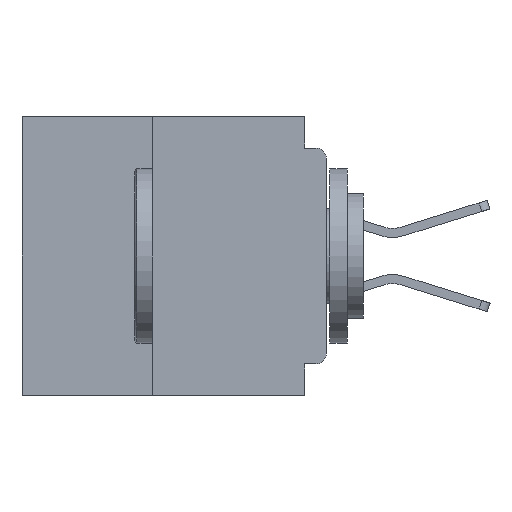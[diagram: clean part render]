
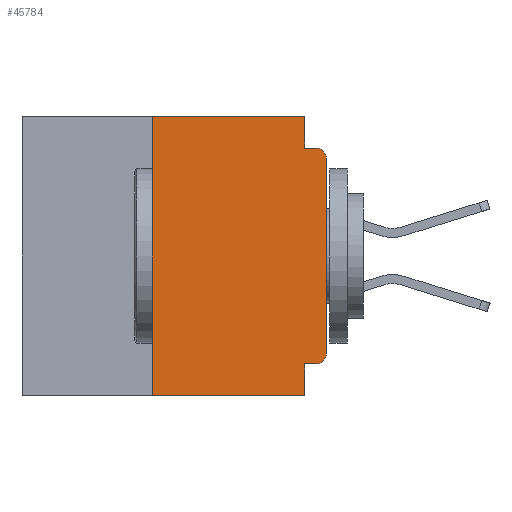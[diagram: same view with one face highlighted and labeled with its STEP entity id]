
A CAD part, left-side view. The second image highlights one B-rep face of the part: STEP entity #45784.
In plain terms, the highlighted planar face has unit normal (-1, 0, 0).
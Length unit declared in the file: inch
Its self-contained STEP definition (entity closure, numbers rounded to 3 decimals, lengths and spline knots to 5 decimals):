
#815 = VERTEX_POINT ( 'NONE', #24449 ) ;
#2517 = PLANE ( 'NONE',  #50532 ) ;
#2631 = CARTESIAN_POINT ( 'NONE',  ( 0., 0.437, 0. ) ) ;
#3236 = ORIENTED_EDGE ( 'NONE', *, *, #13706, .T. ) ;
#3609 = ORIENTED_EDGE ( 'NONE', *, *, #6461, .T. ) ;
#6225 = CARTESIAN_POINT ( 'NONE',  ( 0., 0.031, -0.355 ) ) ;
#6461 = EDGE_CURVE ( 'NONE', #46812, #25700, #29516, .T. ) ;
#6535 = VECTOR ( 'NONE', #26075, 39.37008 ) ;
#6690 = EDGE_CURVE ( 'NONE', #25700, #815, #55011, .T. ) ;
#6711 = ORIENTED_EDGE ( 'NONE', *, *, #54194, .F. ) ;
#7247 = DIRECTION ( 'NONE',  ( 1., 0., 0. ) ) ;
#7588 = CARTESIAN_POINT ( 'NONE',  ( 0., 0.031, 0. ) ) ;
#7964 = EDGE_CURVE ( 'NONE', #59380, #42239, #56283, .T. ) ;
#8168 = LINE ( 'NONE', #38045, #11101 ) ;
#8232 = VERTEX_POINT ( 'NONE', #23353 ) ;
#8508 = EDGE_LOOP ( 'NONE', ( #3609, #45371, #13263, #25605, #38761, #13714, #18836, #10878, #6711, #3236 ) ) ;
#9701 = CARTESIAN_POINT ( 'NONE',  ( 0., 0.015, -0.355 ) ) ;
#9714 = VECTOR ( 'NONE', #47942, 39.37008 ) ;
#10166 = CARTESIAN_POINT ( 'NONE',  ( 0., 0., -0.34 ) ) ;
#10878 = ORIENTED_EDGE ( 'NONE', *, *, #47518, .F. ) ;
#11101 = VECTOR ( 'NONE', #42735, 39.37008 ) ;
#12724 = DIRECTION ( 'NONE',  ( 0., -1., 0. ) ) ;
#13263 = ORIENTED_EDGE ( 'NONE', *, *, #47075, .F. ) ;
#13706 = EDGE_CURVE ( 'NONE', #50700, #46812, #15067, .T. ) ;
#13714 = ORIENTED_EDGE ( 'NONE', *, *, #55266, .F. ) ;
#15067 = CIRCLE ( 'NONE', #31527, 0.015 ) ;
#15524 = CARTESIAN_POINT ( 'NONE',  ( 0., 0., 0. ) ) ;
#16374 = CARTESIAN_POINT ( 'NONE',  ( 0., 0., -0.06 ) ) ;
#17117 = LINE ( 'NONE', #38011, #28136 ) ;
#18836 = ORIENTED_EDGE ( 'NONE', *, *, #40771, .T. ) ;
#21258 = CARTESIAN_POINT ( 'NONE',  ( 0., 0.031, -0.045 ) ) ;
#21298 = CARTESIAN_POINT ( 'NONE',  ( 0., 0.031, -0.4 ) ) ;
#22280 = LINE ( 'NONE', #26181, #58054 ) ;
#23353 = CARTESIAN_POINT ( 'NONE',  ( 0., 0.25, -0.4 ) ) ;
#24449 = CARTESIAN_POINT ( 'NONE',  ( 0., 0.015, -0.045 ) ) ;
#24687 = CARTESIAN_POINT ( 'NONE',  ( 0., 0.031, -0.4 ) ) ;
#25013 = DIRECTION ( 'NONE',  ( 0., 0., 1. ) ) ;
#25605 = ORIENTED_EDGE ( 'NONE', *, *, #27422, .F. ) ;
#25700 = VERTEX_POINT ( 'NONE', #16374 ) ;
#26075 = DIRECTION ( 'NONE',  ( 0., -1., 0. ) ) ;
#26181 = CARTESIAN_POINT ( 'NONE',  ( 0., 0., -0.045 ) ) ;
#26637 = DIRECTION ( 'NONE',  ( -1., 0., 0. ) ) ;
#26736 = DIRECTION ( 'NONE',  ( -1., 0., 0. ) ) ;
#27422 = EDGE_CURVE ( 'NONE', #42239, #50323, #58812, .T. ) ;
#28136 = VECTOR ( 'NONE', #28629, 39.37008 ) ;
#28629 = DIRECTION ( 'NONE',  ( 0., 1., 0. ) ) ;
#29516 = LINE ( 'NONE', #15524, #52818 ) ;
#31527 = AXIS2_PLACEMENT_3D ( 'NONE', #54646, #26736, #59368 ) ;
#35241 = LINE ( 'NONE', #50153, #57084 ) ;
#35478 = VECTOR ( 'NONE', #40378, 39.37008 ) ;
#38011 = CARTESIAN_POINT ( 'NONE',  ( 0., 0., -0.355 ) ) ;
#38045 = CARTESIAN_POINT ( 'NONE',  ( 0., 0.25, -0.4 ) ) ;
#38761 = ORIENTED_EDGE ( 'NONE', *, *, #7964, .F. ) ;
#40031 = DIRECTION ( 'NONE',  ( 0., 0., -1. ) ) ;
#40378 = DIRECTION ( 'NONE',  ( 0., 0., -1. ) ) ;
#40771 = EDGE_CURVE ( 'NONE', #8232, #45145, #35241, .T. ) ;
#42239 = VERTEX_POINT ( 'NONE', #50793 ) ;
#42735 = DIRECTION ( 'NONE',  ( 0., 0., 1. ) ) ;
#44338 = CARTESIAN_POINT ( 'NONE',  ( 0., 0.437, 0. ) ) ;
#45145 = VERTEX_POINT ( 'NONE', #21298 ) ;
#45371 = ORIENTED_EDGE ( 'NONE', *, *, #6690, .T. ) ;
#45784 = ADVANCED_FACE ( 'NONE', ( #45848 ), #2517, .F. ) ;
#45848 = FACE_OUTER_BOUND ( 'NONE', #8508, .T. ) ;
#46812 = VERTEX_POINT ( 'NONE', #10166 ) ;
#47075 = EDGE_CURVE ( 'NONE', #50323, #815, #22280, .T. ) ;
#47518 = EDGE_CURVE ( 'NONE', #59819, #45145, #59498, .T. ) ;
#47942 = DIRECTION ( 'NONE',  ( 0., 0., -1. ) ) ;
#49414 = DIRECTION ( 'NONE',  ( 0., -1., 0. ) ) ;
#49667 = CARTESIAN_POINT ( 'NONE',  ( 0., 0.25, 0. ) ) ;
#50153 = CARTESIAN_POINT ( 'NONE',  ( 0., 0.437, -0.4 ) ) ;
#50323 = VERTEX_POINT ( 'NONE', #21258 ) ;
#50532 = AXIS2_PLACEMENT_3D ( 'NONE', #44338, #7247, #40031 ) ;
#50700 = VERTEX_POINT ( 'NONE', #9701 ) ;
#50793 = CARTESIAN_POINT ( 'NONE',  ( 0., 0.031, 0. ) ) ;
#52818 = VECTOR ( 'NONE', #25013, 39.37008 ) ;
#54194 = EDGE_CURVE ( 'NONE', #50700, #59819, #17117, .T. ) ;
#54533 = CARTESIAN_POINT ( 'NONE',  ( 0., 0.015, -0.06 ) ) ;
#54646 = CARTESIAN_POINT ( 'NONE',  ( 0., 0.015, -0.34 ) ) ;
#55011 = CIRCLE ( 'NONE', #56224, 0.015 ) ;
#55266 = EDGE_CURVE ( 'NONE', #8232, #59380, #8168, .T. ) ;
#56224 = AXIS2_PLACEMENT_3D ( 'NONE', #54533, #26637, #59273 ) ;
#56283 = LINE ( 'NONE', #2631, #6535 ) ;
#57084 = VECTOR ( 'NONE', #12724, 39.37008 ) ;
#58054 = VECTOR ( 'NONE', #49414, 39.37008 ) ;
#58812 = LINE ( 'NONE', #7588, #35478 ) ;
#59273 = DIRECTION ( 'NONE',  ( 0., 0., -1. ) ) ;
#59368 = DIRECTION ( 'NONE',  ( 0., 0., -1. ) ) ;
#59380 = VERTEX_POINT ( 'NONE', #49667 ) ;
#59498 = LINE ( 'NONE', #24687, #9714 ) ;
#59819 = VERTEX_POINT ( 'NONE', #6225 ) ;
